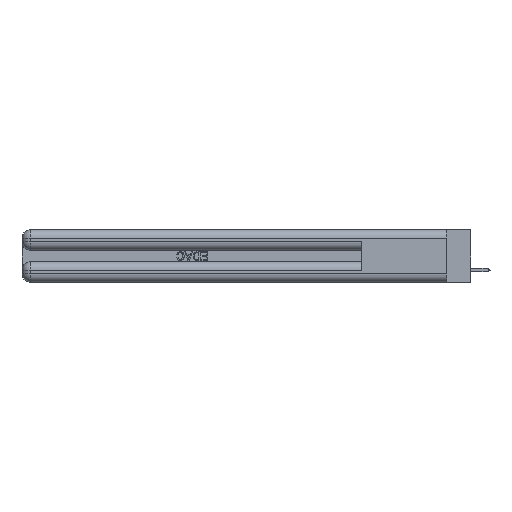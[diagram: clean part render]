
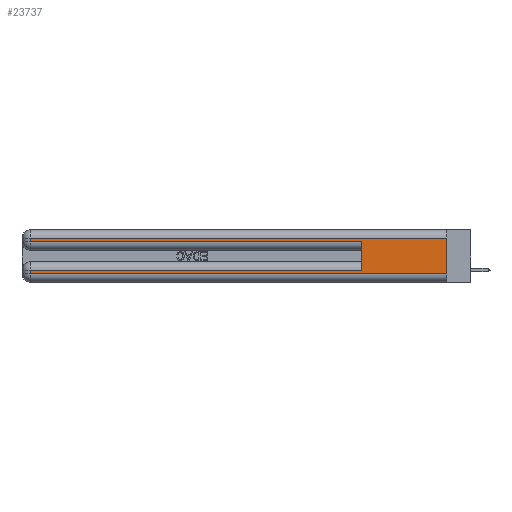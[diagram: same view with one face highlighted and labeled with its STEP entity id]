
A CAD part, left-side view. The second image highlights one B-rep face of the part: STEP entity #23737.
In plain terms, the highlighted planar face has unit normal (-1, 0, 0).
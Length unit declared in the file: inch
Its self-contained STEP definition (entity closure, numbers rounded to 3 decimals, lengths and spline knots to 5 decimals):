
#991 = ORIENTED_EDGE ( 'NONE', *, *, #44154, .T. ) ;
#1463 = CARTESIAN_POINT ( 'NONE',  ( 0., 0., 0.085 ) ) ;
#2692 = EDGE_LOOP ( 'NONE', ( #23938, #6057, #8459, #991, #17520, #53035, #12825, #40606 ) ) ;
#2770 = DIRECTION ( 'NONE',  ( 0., 0., 1. ) ) ;
#3137 = CARTESIAN_POINT ( 'NONE',  ( 0., 0.6, 0.085 ) ) ;
#3440 = EDGE_CURVE ( 'NONE', #25624, #24147, #29677, .T. ) ;
#4738 = VECTOR ( 'NONE', #15391, 39.37008 ) ;
#5352 = LINE ( 'NONE', #9190, #40786 ) ;
#6057 = ORIENTED_EDGE ( 'NONE', *, *, #17176, .T. ) ;
#6606 = CARTESIAN_POINT ( 'NONE',  ( 0., 0., 0.37 ) ) ;
#7071 = CARTESIAN_POINT ( 'NONE',  ( 0., 2.94, 0.37 ) ) ;
#8459 = ORIENTED_EDGE ( 'NONE', *, *, #8935, .T. ) ;
#8935 = EDGE_CURVE ( 'NONE', #27498, #13949, #29315, .T. ) ;
#9190 = CARTESIAN_POINT ( 'NONE',  ( 0., 0., 0.285 ) ) ;
#10231 = VECTOR ( 'NONE', #39690, 39.37008 ) ;
#11406 = VERTEX_POINT ( 'NONE', #49443 ) ;
#12825 = ORIENTED_EDGE ( 'NONE', *, *, #13088, .T. ) ;
#13088 = EDGE_CURVE ( 'NONE', #52978, #25624, #48430, .T. ) ;
#13949 = VERTEX_POINT ( 'NONE', #19894 ) ;
#14219 = CARTESIAN_POINT ( 'NONE',  ( 0., 0., 0.31 ) ) ;
#15288 = DIRECTION ( 'NONE',  ( 0., 1., 0. ) ) ;
#15321 = EDGE_CURVE ( 'NONE', #41780, #52978, #51171, .T. ) ;
#15391 = DIRECTION ( 'NONE',  ( 0., -1., 0. ) ) ;
#17030 = CARTESIAN_POINT ( 'NONE',  ( 0., 0., 0.37 ) ) ;
#17176 = EDGE_CURVE ( 'NONE', #40357, #27498, #27517, .T. ) ;
#17520 = ORIENTED_EDGE ( 'NONE', *, *, #20441, .F. ) ;
#19894 = CARTESIAN_POINT ( 'NONE',  ( 0., 2.94, 0.285 ) ) ;
#20086 = CARTESIAN_POINT ( 'NONE',  ( 0., 0., 0.31 ) ) ;
#20441 = EDGE_CURVE ( 'NONE', #41780, #11406, #35658, .T. ) ;
#21255 = DIRECTION ( 'NONE',  ( 1., 0., 0. ) ) ;
#21607 = VECTOR ( 'NONE', #15288, 39.37008 ) ;
#23737 = ADVANCED_FACE ( 'NONE', ( #39278 ), #54205, .F. ) ;
#23938 = ORIENTED_EDGE ( 'NONE', *, *, #41668, .F. ) ;
#24147 = VERTEX_POINT ( 'NONE', #47015 ) ;
#24615 = LINE ( 'NONE', #6606, #46214 ) ;
#25486 = DIRECTION ( 'NONE',  ( 0., 0., -1. ) ) ;
#25624 = VERTEX_POINT ( 'NONE', #39702 ) ;
#27498 = VERTEX_POINT ( 'NONE', #31303 ) ;
#27517 = LINE ( 'NONE', #20086, #21607 ) ;
#29315 = LINE ( 'NONE', #7071, #10231 ) ;
#29677 = LINE ( 'NONE', #40698, #4738 ) ;
#29755 = DIRECTION ( 'NONE',  ( 0., -1., 0. ) ) ;
#31303 = CARTESIAN_POINT ( 'NONE',  ( 0., 2.94, 0.31 ) ) ;
#35658 = LINE ( 'NONE', #36514, #42822 ) ;
#35975 = DIRECTION ( 'NONE',  ( 0., 0., -1. ) ) ;
#36514 = CARTESIAN_POINT ( 'NONE',  ( 0., 0.6, 0.145 ) ) ;
#36781 = CARTESIAN_POINT ( 'NONE',  ( 0., 2.94, 0.085 ) ) ;
#38641 = AXIS2_PLACEMENT_3D ( 'NONE', #17030, #21255, #25486 ) ;
#39215 = VECTOR ( 'NONE', #49775, 39.37008 ) ;
#39278 = FACE_OUTER_BOUND ( 'NONE', #2692, .T. ) ;
#39690 = DIRECTION ( 'NONE',  ( 0., 0., -1. ) ) ;
#39702 = CARTESIAN_POINT ( 'NONE',  ( 0., 2.94, 0.06 ) ) ;
#40104 = VECTOR ( 'NONE', #47774, 39.37008 ) ;
#40357 = VERTEX_POINT ( 'NONE', #14219 ) ;
#40488 = CARTESIAN_POINT ( 'NONE',  ( 0., 2.94, 0.37 ) ) ;
#40606 = ORIENTED_EDGE ( 'NONE', *, *, #3440, .T. ) ;
#40698 = CARTESIAN_POINT ( 'NONE',  ( 0., 0., 0.06 ) ) ;
#40786 = VECTOR ( 'NONE', #29755, 39.37008 ) ;
#41668 = EDGE_CURVE ( 'NONE', #40357, #24147, #24615, .T. ) ;
#41780 = VERTEX_POINT ( 'NONE', #3137 ) ;
#42822 = VECTOR ( 'NONE', #2770, 39.37008 ) ;
#44154 = EDGE_CURVE ( 'NONE', #13949, #11406, #5352, .T. ) ;
#46214 = VECTOR ( 'NONE', #35975, 39.37008 ) ;
#47015 = CARTESIAN_POINT ( 'NONE',  ( 0., 0., 0.06 ) ) ;
#47774 = DIRECTION ( 'NONE',  ( 0., 1., 0. ) ) ;
#48430 = LINE ( 'NONE', #40488, #39215 ) ;
#49443 = CARTESIAN_POINT ( 'NONE',  ( 0., 0.6, 0.285 ) ) ;
#49775 = DIRECTION ( 'NONE',  ( 0., 0., -1. ) ) ;
#51171 = LINE ( 'NONE', #1463, #40104 ) ;
#52978 = VERTEX_POINT ( 'NONE', #36781 ) ;
#53035 = ORIENTED_EDGE ( 'NONE', *, *, #15321, .T. ) ;
#54205 = PLANE ( 'NONE',  #38641 ) ;
